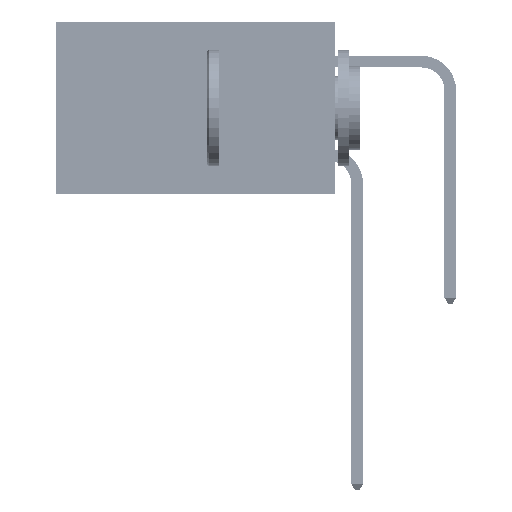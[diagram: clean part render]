
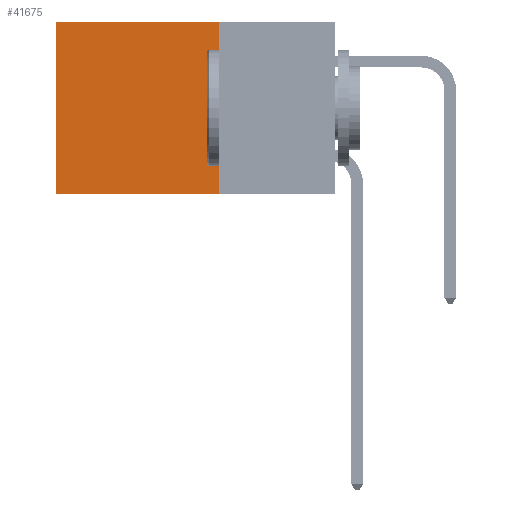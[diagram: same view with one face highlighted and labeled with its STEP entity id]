
A CAD part, left-side view. The second image highlights one B-rep face of the part: STEP entity #41675.
In plain terms, the highlighted planar face has unit normal (-1, 0, 0).
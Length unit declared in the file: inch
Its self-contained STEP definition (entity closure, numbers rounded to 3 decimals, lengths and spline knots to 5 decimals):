
#800 = DIRECTION ( 'NONE',  ( 0., 0., -1. ) ) ;
#1544 = CARTESIAN_POINT ( 'NONE',  ( 0.2875, 0.25, -0.37 ) ) ;
#5472 = ORIENTED_EDGE ( 'NONE', *, *, #16285, .T. ) ;
#5907 = EDGE_CURVE ( 'NONE', #14664, #7073, #24706, .T. ) ;
#6678 = LINE ( 'NONE', #23583, #18977 ) ;
#7073 = VERTEX_POINT ( 'NONE', #43193 ) ;
#7626 = VECTOR ( 'NONE', #46213, 39.37008 ) ;
#7633 = CARTESIAN_POINT ( 'NONE',  ( 0.2875, 0.25, 0. ) ) ;
#13245 = VERTEX_POINT ( 'NONE', #7633 ) ;
#13380 = AXIS2_PLACEMENT_3D ( 'NONE', #33436, #44721, #19703 ) ;
#13571 = DIRECTION ( 'NONE',  ( 0., 1., 0. ) ) ;
#14664 = VERTEX_POINT ( 'NONE', #40842 ) ;
#16285 = EDGE_CURVE ( 'NONE', #13245, #42262, #6678, .T. ) ;
#18835 = LINE ( 'NONE', #39162, #7626 ) ;
#18977 = VECTOR ( 'NONE', #13571, 39.37008 ) ;
#19017 = LINE ( 'NONE', #22196, #26292 ) ;
#19703 = DIRECTION ( 'NONE',  ( 0., 0., -1. ) ) ;
#21015 = EDGE_CURVE ( 'NONE', #42262, #7073, #19017, .T. ) ;
#22196 = CARTESIAN_POINT ( 'NONE',  ( 0.2875, 0.6, 0. ) ) ;
#23046 = ORIENTED_EDGE ( 'NONE', *, *, #5907, .F. ) ;
#23234 = ORIENTED_EDGE ( 'NONE', *, *, #21015, .T. ) ;
#23583 = CARTESIAN_POINT ( 'NONE',  ( 0.2875, 0.25, 0. ) ) ;
#24706 = LINE ( 'NONE', #1544, #45436 ) ;
#25878 = EDGE_LOOP ( 'NONE', ( #23234, #23046, #32279, #5472 ) ) ;
#26292 = VECTOR ( 'NONE', #800, 39.37008 ) ;
#26547 = DIRECTION ( 'NONE',  ( 0., 1., 0. ) ) ;
#30670 = EDGE_CURVE ( 'NONE', #13245, #14664, #18835, .T. ) ;
#32279 = ORIENTED_EDGE ( 'NONE', *, *, #30670, .F. ) ;
#33436 = CARTESIAN_POINT ( 'NONE',  ( 0.2875, 0.25, 0. ) ) ;
#37103 = FACE_OUTER_BOUND ( 'NONE', #25878, .T. ) ;
#39162 = CARTESIAN_POINT ( 'NONE',  ( 0.2875, 0.25, 0. ) ) ;
#40842 = CARTESIAN_POINT ( 'NONE',  ( 0.2875, 0.25, -0.37 ) ) ;
#40934 = CARTESIAN_POINT ( 'NONE',  ( 0.2875, 0.6, 0. ) ) ;
#41152 = PLANE ( 'NONE',  #13380 ) ;
#41675 = ADVANCED_FACE ( 'NONE', ( #37103 ), #41152, .F. ) ;
#42262 = VERTEX_POINT ( 'NONE', #40934 ) ;
#43193 = CARTESIAN_POINT ( 'NONE',  ( 0.2875, 0.6, -0.37 ) ) ;
#44721 = DIRECTION ( 'NONE',  ( 1., 0., 0. ) ) ;
#45436 = VECTOR ( 'NONE', #26547, 39.37008 ) ;
#46213 = DIRECTION ( 'NONE',  ( 0., 0., -1. ) ) ;
